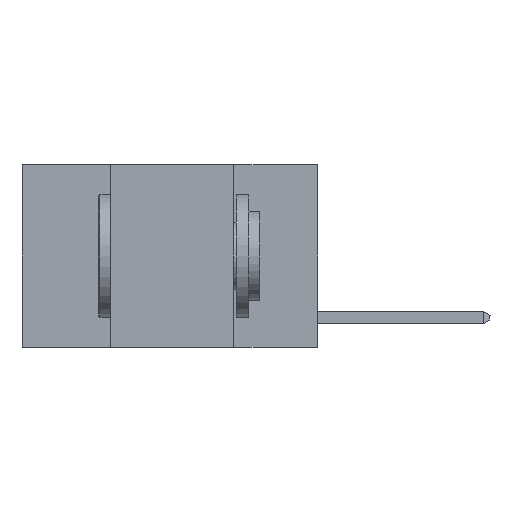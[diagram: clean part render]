
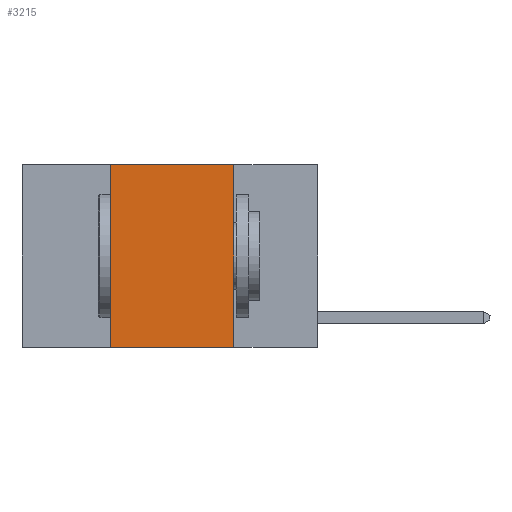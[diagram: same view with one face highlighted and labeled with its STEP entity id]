
A CAD part, left-side view. The second image highlights one B-rep face of the part: STEP entity #3215.
In plain terms, the highlighted planar face has unit normal (-1, 0, 0).
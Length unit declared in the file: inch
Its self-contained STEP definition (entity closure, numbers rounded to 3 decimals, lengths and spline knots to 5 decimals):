
#1300 = AXIS2_PLACEMENT_3D ( 'NONE', #11079, #12957, #4673 ) ;
#1362 = VECTOR ( 'NONE', #6476, 39.37008 ) ;
#1821 = LINE ( 'NONE', #11568, #13156 ) ;
#1904 = EDGE_CURVE ( 'NONE', #4923, #6918, #1821, .T. ) ;
#1920 = VECTOR ( 'NONE', #7023, 39.37008 ) ;
#2599 = ORIENTED_EDGE ( 'NONE', *, *, #3942, .F. ) ;
#2630 = EDGE_LOOP ( 'NONE', ( #2599, #8502, #9923, #3590 ) ) ;
#3215 = ADVANCED_FACE ( 'NONE', ( #7631 ), #13440, .F. ) ;
#3590 = ORIENTED_EDGE ( 'NONE', *, *, #4022, .T. ) ;
#3942 = EDGE_CURVE ( 'NONE', #6918, #5303, #8749, .T. ) ;
#3967 = EDGE_CURVE ( 'NONE', #13436, #4923, #13228, .T. ) ;
#4022 = EDGE_CURVE ( 'NONE', #13436, #5303, #10540, .T. ) ;
#4673 = DIRECTION ( 'NONE',  ( 0., 0., -1. ) ) ;
#4923 = VERTEX_POINT ( 'NONE', #9545 ) ;
#5303 = VERTEX_POINT ( 'NONE', #14250 ) ;
#6405 = CARTESIAN_POINT ( 'NONE',  ( 0., 0.6, -0.37 ) ) ;
#6476 = DIRECTION ( 'NONE',  ( 0., -1., 0. ) ) ;
#6918 = VERTEX_POINT ( 'NONE', #11992 ) ;
#7023 = DIRECTION ( 'NONE',  ( 0., 0., 1. ) ) ;
#7090 = CARTESIAN_POINT ( 'NONE',  ( 0., 0.42, 0. ) ) ;
#7631 = FACE_OUTER_BOUND ( 'NONE', #2630, .T. ) ;
#7785 = DIRECTION ( 'NONE',  ( 0., 0., -1. ) ) ;
#7837 = CARTESIAN_POINT ( 'NONE',  ( 0., 0.17, 0. ) ) ;
#8069 = CARTESIAN_POINT ( 'NONE',  ( 0., 0.42, -0.37 ) ) ;
#8502 = ORIENTED_EDGE ( 'NONE', *, *, #1904, .F. ) ;
#8749 = LINE ( 'NONE', #7837, #13830 ) ;
#9545 = CARTESIAN_POINT ( 'NONE',  ( 0., 0.42, 0. ) ) ;
#9923 = ORIENTED_EDGE ( 'NONE', *, *, #3967, .F. ) ;
#10540 = LINE ( 'NONE', #6405, #1362 ) ;
#11079 = CARTESIAN_POINT ( 'NONE',  ( 0., 0.6, 0. ) ) ;
#11244 = DIRECTION ( 'NONE',  ( 0., -1., 0. ) ) ;
#11568 = CARTESIAN_POINT ( 'NONE',  ( 0., 0.6, 0. ) ) ;
#11992 = CARTESIAN_POINT ( 'NONE',  ( 0., 0.17, 0. ) ) ;
#12957 = DIRECTION ( 'NONE',  ( 1., 0., 0. ) ) ;
#13156 = VECTOR ( 'NONE', #11244, 39.37008 ) ;
#13228 = LINE ( 'NONE', #7090, #1920 ) ;
#13436 = VERTEX_POINT ( 'NONE', #8069 ) ;
#13440 = PLANE ( 'NONE',  #1300 ) ;
#13830 = VECTOR ( 'NONE', #7785, 39.37008 ) ;
#14250 = CARTESIAN_POINT ( 'NONE',  ( 0., 0.17, -0.37 ) ) ;
